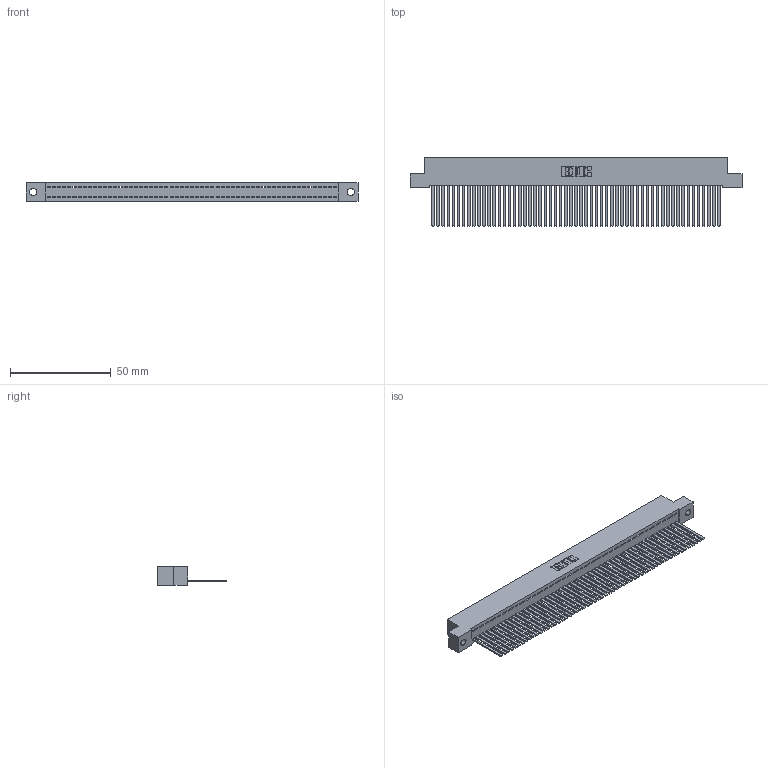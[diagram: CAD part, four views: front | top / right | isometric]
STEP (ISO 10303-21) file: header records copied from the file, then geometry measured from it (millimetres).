
FILE_DESCRIPTION (( 'STEP AP203' ), '1' );
FILE_NAME ('392-057-544-102.STEP', '2018-08-17T15:27:03', ( '' ), ( '' ), 'SwSTEP 2.0', 'SolidWorks 2016', '' );
FILE_SCHEMA (( 'CONFIG_CONTROL_DESIGN' ));
Length unit declared in the file: inch
Products named in the file (3): 392-057-544-102; 342 Part_.128 Slot; 345-292-001_345-293-144
Assembly tree (58 placements, depth 2):
  392-057-544-102
    342 Part_.128 Slot
    345-292-001_345-293-144  x57
Bounding box: 165.1 x 34.3 x 9.4 mm (x, y, z)
Volume: 15139.2 mm3; surface area: 24149.7 mm2
Topology: 58 solids, 58 shells, 3078 faces, 9317 edges, 6134 vertices
Faces by surface type: plane 2236, cylinder 842
Entity records: 32725 total; most frequent: CARTESIAN_POINT 5649, ORIENTED_EDGE 5642, DIRECTION 4731, EDGE_CURVE 2821, VECTOR 2697, LINE 2697, VERTEX_POINT 1878, AXIS2_PLACEMENT_3D 1017
